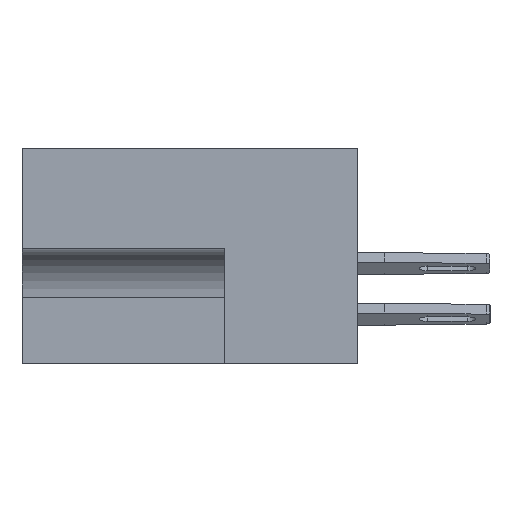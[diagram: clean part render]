
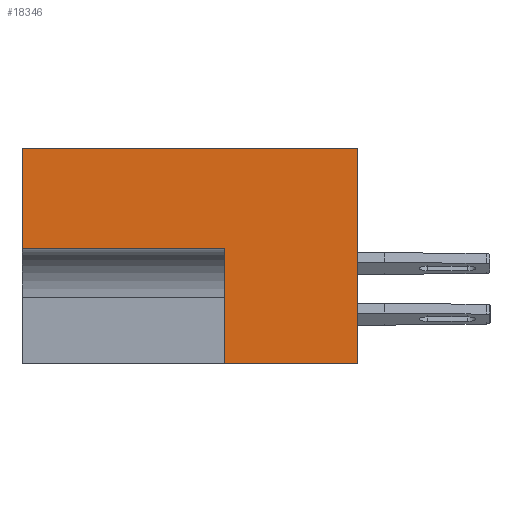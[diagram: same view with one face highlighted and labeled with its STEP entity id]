
A CAD part, left-side view. The second image highlights one B-rep face of the part: STEP entity #18346.
In plain terms, the highlighted planar face has unit normal (-1, 0, 0).
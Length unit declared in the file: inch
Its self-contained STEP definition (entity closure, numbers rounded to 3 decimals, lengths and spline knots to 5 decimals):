
#332 = CARTESIAN_POINT ( 'NONE',  ( 0., 0.828, 0. ) ) ;
#1055 = VECTOR ( 'NONE', #15506, 39.37008 ) ;
#1156 = EDGE_CURVE ( 'NONE', #26099, #6992, #14472, .T. ) ;
#2303 = ORIENTED_EDGE ( 'NONE', *, *, #9499, .F. ) ;
#3147 = VERTEX_POINT ( 'NONE', #15337 ) ;
#4503 = VERTEX_POINT ( 'NONE', #7907 ) ;
#4698 = VECTOR ( 'NONE', #12998, 39.37008 ) ;
#4791 = ORIENTED_EDGE ( 'NONE', *, *, #10660, .T. ) ;
#5893 = CARTESIAN_POINT ( 'NONE',  ( 0., 0., 0. ) ) ;
#5970 = EDGE_CURVE ( 'NONE', #26097, #6407, #13494, .T. ) ;
#6014 = ORIENTED_EDGE ( 'NONE', *, *, #5970, .F. ) ;
#6407 = VERTEX_POINT ( 'NONE', #332 ) ;
#6807 = CARTESIAN_POINT ( 'NONE',  ( 0., 0., -0.531 ) ) ;
#6992 = VERTEX_POINT ( 'NONE', #6807 ) ;
#7907 = CARTESIAN_POINT ( 'NONE',  ( 0., 0.328, -0.248 ) ) ;
#8018 = ORIENTED_EDGE ( 'NONE', *, *, #1156, .T. ) ;
#8108 = ORIENTED_EDGE ( 'NONE', *, *, #22730, .F. ) ;
#8682 = CARTESIAN_POINT ( 'NONE',  ( 0., 0.828, -0.248 ) ) ;
#9499 = EDGE_CURVE ( 'NONE', #26099, #4503, #25720, .T. ) ;
#9820 = DIRECTION ( 'NONE',  ( 0., 0., 1. ) ) ;
#9838 = FACE_OUTER_BOUND ( 'NONE', #16432, .T. ) ;
#9879 = VECTOR ( 'NONE', #9820, 39.37008 ) ;
#9991 = CARTESIAN_POINT ( 'NONE',  ( 0., 0.828, 0. ) ) ;
#10021 = DIRECTION ( 'NONE',  ( 0., -1., 0. ) ) ;
#10660 = EDGE_CURVE ( 'NONE', #6992, #3147, #25765, .T. ) ;
#11181 = VECTOR ( 'NONE', #10021, 39.37008 ) ;
#11280 = PLANE ( 'NONE',  #11334 ) ;
#11334 = AXIS2_PLACEMENT_3D ( 'NONE', #19591, #23866, #15284 ) ;
#12720 = CARTESIAN_POINT ( 'NONE',  ( 0., 0.453, -0.531 ) ) ;
#12998 = DIRECTION ( 'NONE',  ( 0., -1., 0. ) ) ;
#13145 = LINE ( 'NONE', #26650, #11181 ) ;
#13494 = LINE ( 'NONE', #9991, #9879 ) ;
#14472 = LINE ( 'NONE', #12720, #4698 ) ;
#14870 = DIRECTION ( 'NONE',  ( 0., 0., 1. ) ) ;
#15284 = DIRECTION ( 'NONE',  ( 0., 0., -1. ) ) ;
#15337 = CARTESIAN_POINT ( 'NONE',  ( 0., 0., 0. ) ) ;
#15506 = DIRECTION ( 'NONE',  ( 0., 1., 0. ) ) ;
#16432 = EDGE_LOOP ( 'NONE', ( #6014, #8108, #2303, #8018, #4791, #21933 ) ) ;
#18346 = ADVANCED_FACE ( 'NONE', ( #9838 ), #11280, .F. ) ;
#18376 = LINE ( 'NONE', #19447, #1055 ) ;
#19188 = CARTESIAN_POINT ( 'NONE',  ( 0., 0.328, -0.531 ) ) ;
#19447 = CARTESIAN_POINT ( 'NONE',  ( 0., 0.328, -0.248 ) ) ;
#19591 = CARTESIAN_POINT ( 'NONE',  ( 0., 0.453, 0. ) ) ;
#21174 = CARTESIAN_POINT ( 'NONE',  ( 0., 0.328, -0.531 ) ) ;
#21933 = ORIENTED_EDGE ( 'NONE', *, *, #22419, .F. ) ;
#22419 = EDGE_CURVE ( 'NONE', #6407, #3147, #13145, .T. ) ;
#22609 = DIRECTION ( 'NONE',  ( 0., 0., 1. ) ) ;
#22730 = EDGE_CURVE ( 'NONE', #4503, #26097, #18376, .T. ) ;
#23784 = VECTOR ( 'NONE', #22609, 39.37008 ) ;
#23866 = DIRECTION ( 'NONE',  ( 1., 0., 0. ) ) ;
#25055 = VECTOR ( 'NONE', #14870, 39.37008 ) ;
#25720 = LINE ( 'NONE', #21174, #25055 ) ;
#25765 = LINE ( 'NONE', #5893, #23784 ) ;
#26097 = VERTEX_POINT ( 'NONE', #8682 ) ;
#26099 = VERTEX_POINT ( 'NONE', #19188 ) ;
#26650 = CARTESIAN_POINT ( 'NONE',  ( 0., 0.453, 0. ) ) ;
